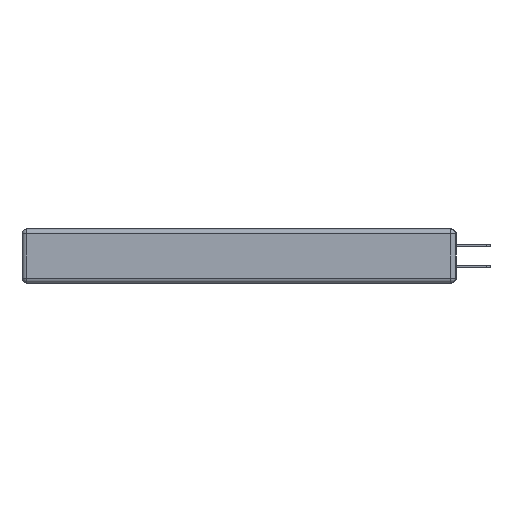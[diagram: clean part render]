
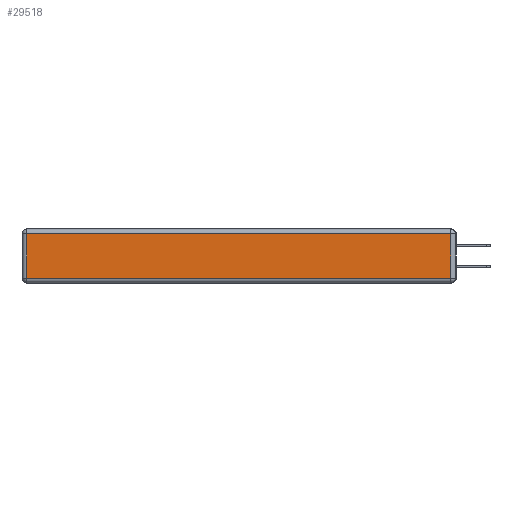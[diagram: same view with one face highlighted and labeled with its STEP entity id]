
A CAD part, left-side view. The second image highlights one B-rep face of the part: STEP entity #29518.
In plain terms, the highlighted planar face has unit normal (-1, 0, 0).
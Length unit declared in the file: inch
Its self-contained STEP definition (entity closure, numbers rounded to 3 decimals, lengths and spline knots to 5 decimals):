
#358 = EDGE_LOOP ( 'NONE', ( #22744, #5151, #29989, #11801 ) ) ;
#1249 = CARTESIAN_POINT ( 'NONE',  ( 0., 2.75, -0.03 ) ) ;
#1670 = DIRECTION ( 'NONE',  ( 0., 1., 0. ) ) ;
#1778 = EDGE_CURVE ( 'NONE', #26069, #24410, #20449, .T. ) ;
#2602 = CARTESIAN_POINT ( 'NONE',  ( 0., 0., -0.313 ) ) ;
#3594 = CARTESIAN_POINT ( 'NONE',  ( 0., 0.03, -0.03 ) ) ;
#3719 = VECTOR ( 'NONE', #1670, 39.37008 ) ;
#5151 = ORIENTED_EDGE ( 'NONE', *, *, #22456, .T. ) ;
#5720 = VECTOR ( 'NONE', #27647, 39.37008 ) ;
#6112 = PLANE ( 'NONE',  #29076 ) ;
#6835 = DIRECTION ( 'NONE',  ( 0., 0., 1. ) ) ;
#6845 = LINE ( 'NONE', #15675, #5720 ) ;
#7421 = CARTESIAN_POINT ( 'NONE',  ( 0., 2.72, -0.313 ) ) ;
#7427 = LINE ( 'NONE', #2602, #16757 ) ;
#8066 = DIRECTION ( 'NONE',  ( 0., 0., -1. ) ) ;
#8736 = LINE ( 'NONE', #12846, #16193 ) ;
#9386 = CARTESIAN_POINT ( 'NONE',  ( 0., 0.03, -0.313 ) ) ;
#9785 = VERTEX_POINT ( 'NONE', #9386 ) ;
#10959 = CARTESIAN_POINT ( 'NONE',  ( 0., 2.72, -0.03 ) ) ;
#11618 = DIRECTION ( 'NONE',  ( -1., 0., 0. ) ) ;
#11801 = ORIENTED_EDGE ( 'NONE', *, *, #18369, .T. ) ;
#12259 = DIRECTION ( 'NONE',  ( 0., -1., 0. ) ) ;
#12846 = CARTESIAN_POINT ( 'NONE',  ( 0., 2.72, -0.343 ) ) ;
#15675 = CARTESIAN_POINT ( 'NONE',  ( 0., 0.03, -0.343 ) ) ;
#16193 = VECTOR ( 'NONE', #8066, 39.37008 ) ;
#16757 = VECTOR ( 'NONE', #12259, 39.37008 ) ;
#18369 = EDGE_CURVE ( 'NONE', #24410, #18891, #8736, .T. ) ;
#18891 = VERTEX_POINT ( 'NONE', #7421 ) ;
#20449 = LINE ( 'NONE', #1249, #3719 ) ;
#21402 = FACE_OUTER_BOUND ( 'NONE', #358, .T. ) ;
#22456 = EDGE_CURVE ( 'NONE', #9785, #26069, #6845, .T. ) ;
#22744 = ORIENTED_EDGE ( 'NONE', *, *, #27723, .T. ) ;
#24410 = VERTEX_POINT ( 'NONE', #10959 ) ;
#25229 = CARTESIAN_POINT ( 'NONE',  ( 0., 0., -0.343 ) ) ;
#26069 = VERTEX_POINT ( 'NONE', #3594 ) ;
#27647 = DIRECTION ( 'NONE',  ( 0., 0., 1. ) ) ;
#27723 = EDGE_CURVE ( 'NONE', #18891, #9785, #7427, .T. ) ;
#29076 = AXIS2_PLACEMENT_3D ( 'NONE', #25229, #11618, #6835 ) ;
#29518 = ADVANCED_FACE ( 'NONE', ( #21402 ), #6112, .T. ) ;
#29989 = ORIENTED_EDGE ( 'NONE', *, *, #1778, .T. ) ;
